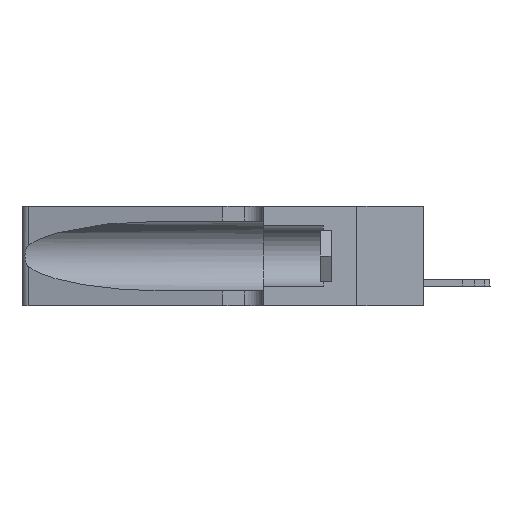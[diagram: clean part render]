
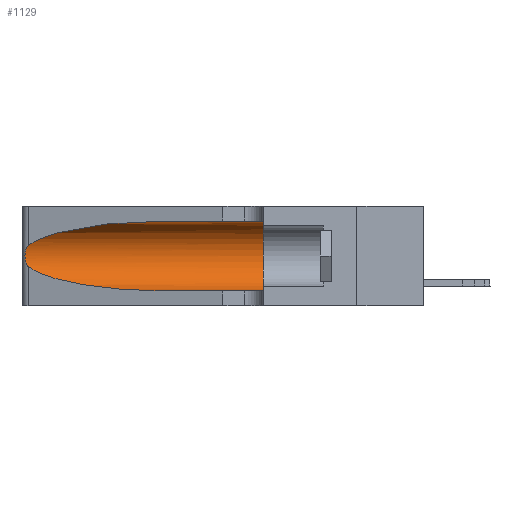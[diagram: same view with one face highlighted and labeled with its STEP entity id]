
A CAD part, left-side view. The second image highlights one B-rep face of the part: STEP entity #1129.
In plain terms, the highlighted cylindrical face has radius 3.308 mm (diameter 6.617 mm), a partial arc.
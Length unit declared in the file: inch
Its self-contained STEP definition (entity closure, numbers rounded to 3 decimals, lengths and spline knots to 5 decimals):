
#900 = CARTESIAN_POINT ( 'NONE',  ( 0.25487, 1.22718, 0.22369 ) ) ;
#940 = CARTESIAN_POINT ( 'NONE',  ( 0.1305, 1.61858, 0.185 ) ) ;
#1116 = CARTESIAN_POINT ( 'NONE',  ( 0.1305, 0.72297, 0.31525 ) ) ;
#1129 = ADVANCED_FACE ( 'NONE', ( #5063 ), #8446, .F. ) ;
#1958 = CARTESIAN_POINT ( 'NONE',  ( 0.25487, 1.22718, 0.14631 ) ) ;
#2099 = AXIS2_PLACEMENT_3D ( 'NONE', #940, #14384, #6208 ) ;
#2236 = EDGE_CURVE ( 'NONE', #19394, #9798, #2392, .T. ) ;
#2392 = B_SPLINE_CURVE_WITH_KNOTS ( 'NONE', 3,
 ( #900, #5565, #15732, #5869, #4059, #17380, #4411, #9474, #2837, #12801, #2765, #2911, #6093, #10994 ),
 .UNSPECIFIED., .F., .F.,
 ( 4, 2, 2, 2, 2, 2, 4 ),
 ( 0., 0.00027, 0.00053, 0.00107, 0.0016, 0.00187, 0.00214 ),
 .UNSPECIFIED. ) ;
#2627 = CARTESIAN_POINT ( 'NONE',  ( 0.1305, 0.72297, 0.31525 ) ) ;
#2703 = CARTESIAN_POINT ( 'NONE',  ( 0.25487, 1.22718, 0.22369 ) ) ;
#2765 = CARTESIAN_POINT ( 'NONE',  ( 0.25789, 1.23486, 0.15765 ) ) ;
#2837 = CARTESIAN_POINT ( 'NONE',  ( 0.26017, 1.23833, 0.17102 ) ) ;
#2911 = CARTESIAN_POINT ( 'NONE',  ( 0.25639, 1.23186, 0.15144 ) ) ;
#4059 = CARTESIAN_POINT ( 'NONE',  ( 0.25854, 1.2359, 0.20912 ) ) ;
#4278 = CARTESIAN_POINT ( 'NONE',  ( 0.2373, 1.15595, 0.28018 ) ) ;
#4411 = CARTESIAN_POINT ( 'NONE',  ( 0.26075, 1.23896, 0.19203 ) ) ;
#4442 = EDGE_CURVE ( 'NONE', #12166, #11646, #16792, .T. ) ;
#4621 = DIRECTION ( 'NONE',  ( 0., 1., 0. ) ) ;
#5063 = FACE_OUTER_BOUND ( 'NONE', #18109, .T. ) ;
#5565 = CARTESIAN_POINT ( 'NONE',  ( 0.25555, 1.22994, 0.2215 ) ) ;
#5667 = CARTESIAN_POINT ( 'NONE',  ( 0.25487, 1.22718, 0.14631 ) ) ;
#5869 = CARTESIAN_POINT ( 'NONE',  ( 0.25787, 1.23484, 0.2124 ) ) ;
#5948 = CARTESIAN_POINT ( 'NONE',  ( 0.18966, 0.96281, 0.31525 ) ) ;
#6093 = CARTESIAN_POINT ( 'NONE',  ( 0.25555, 1.22993, 0.14849 ) ) ;
#6208 = DIRECTION ( 'NONE',  ( 0., 0., -1. ) ) ;
#6311 = EDGE_CURVE ( 'NONE', #12266, #19394, #8343, .T. ) ;
#7285 = CARTESIAN_POINT ( 'NONE',  ( 0.1305, 0.35, 0.31525 ) ) ;
#7495 = CARTESIAN_POINT ( 'NONE',  ( 0.1305, 0.72297, 0.05475 ) ) ;
#7782 = CARTESIAN_POINT ( 'NONE',  ( 0.1305, 1.61858, 0.31525 ) ) ;
#8343 =( BOUNDED_CURVE ( )  B_SPLINE_CURVE ( 3, ( #2627, #5948, #4278, #2703 ),
 .UNSPECIFIED., .F., .T. ) 
 B_SPLINE_CURVE_WITH_KNOTS ( ( 4, 4 ),
 ( 1.5708, 2.84003 ),
 .UNSPECIFIED. ) 
 CURVE ( )  GEOMETRIC_REPRESENTATION_ITEM ( )  RATIONAL_B_SPLINE_CURVE ( ( 1., 0.87, 0.87, 1. ) ) 
 REPRESENTATION_ITEM ( '' )  );
#8446 = CYLINDRICAL_SURFACE ( 'NONE', #2099, 0.13025 ) ;
#9414 =( BOUNDED_CURVE ( )  B_SPLINE_CURVE ( 3, ( #5667, #12314, #10872, #7495 ),
 .UNSPECIFIED., .F., .T. ) 
 B_SPLINE_CURVE_WITH_KNOTS ( ( 4, 4 ),
 ( 3.44316, 4.71239 ),
 .UNSPECIFIED. ) 
 CURVE ( )  GEOMETRIC_REPRESENTATION_ITEM ( )  RATIONAL_B_SPLINE_CURVE ( ( 1., 0.87, 0.87, 1. ) ) 
 REPRESENTATION_ITEM ( '' )  );
#9474 = CARTESIAN_POINT ( 'NONE',  ( 0.26075, 1.23896, 0.178 ) ) ;
#9798 = VERTEX_POINT ( 'NONE', #1958 ) ;
#10486 = ORIENTED_EDGE ( 'NONE', *, *, #16818, .F. ) ;
#10689 = CARTESIAN_POINT ( 'NONE',  ( 0.1305, 1.61858, 0.05475 ) ) ;
#10872 = CARTESIAN_POINT ( 'NONE',  ( 0.18966, 0.96281, 0.05475 ) ) ;
#10994 = CARTESIAN_POINT ( 'NONE',  ( 0.25487, 1.22718, 0.14631 ) ) ;
#11200 = CARTESIAN_POINT ( 'NONE',  ( 0.25487, 1.22718, 0.22369 ) ) ;
#11646 = VERTEX_POINT ( 'NONE', #16860 ) ;
#11823 = VECTOR ( 'NONE', #12001, 39.37008 ) ;
#12001 = DIRECTION ( 'NONE',  ( 0., -1., 0. ) ) ;
#12166 = VERTEX_POINT ( 'NONE', #7285 ) ;
#12266 = VERTEX_POINT ( 'NONE', #1116 ) ;
#12294 = CARTESIAN_POINT ( 'NONE',  ( 0.1305, 0.35, 0.185 ) ) ;
#12314 = CARTESIAN_POINT ( 'NONE',  ( 0.2373, 1.15595, 0.08982 ) ) ;
#12671 = VECTOR ( 'NONE', #17974, 39.37008 ) ;
#12801 = CARTESIAN_POINT ( 'NONE',  ( 0.25856, 1.23593, 0.16098 ) ) ;
#13644 = ORIENTED_EDGE ( 'NONE', *, *, #17878, .T. ) ;
#13728 = ORIENTED_EDGE ( 'NONE', *, *, #16250, .T. ) ;
#14384 = DIRECTION ( 'NONE',  ( 0., -1., 0. ) ) ;
#15189 = CARTESIAN_POINT ( 'NONE',  ( 0.1305, 0.72297, 0.05475 ) ) ;
#15732 = CARTESIAN_POINT ( 'NONE',  ( 0.25639, 1.23184, 0.21858 ) ) ;
#15816 = VERTEX_POINT ( 'NONE', #15189 ) ;
#16250 = EDGE_CURVE ( 'NONE', #9798, #15816, #9414, .T. ) ;
#16486 = AXIS2_PLACEMENT_3D ( 'NONE', #12294, #4621, #20117 ) ;
#16792 = CIRCLE ( 'NONE', #16486, 0.13025 ) ;
#16818 = EDGE_CURVE ( 'NONE', #12266, #12166, #20891, .T. ) ;
#16860 = CARTESIAN_POINT ( 'NONE',  ( 0.1305, 0.35, 0.05475 ) ) ;
#17380 = CARTESIAN_POINT ( 'NONE',  ( 0.26018, 1.23835, 0.19895 ) ) ;
#17878 = EDGE_CURVE ( 'NONE', #15816, #11646, #20578, .T. ) ;
#17974 = DIRECTION ( 'NONE',  ( 0., -1., 0. ) ) ;
#18109 = EDGE_LOOP ( 'NONE', ( #19620, #19354, #13728, #13644, #18591, #10486 ) ) ;
#18591 = ORIENTED_EDGE ( 'NONE', *, *, #4442, .F. ) ;
#19354 = ORIENTED_EDGE ( 'NONE', *, *, #2236, .T. ) ;
#19394 = VERTEX_POINT ( 'NONE', #11200 ) ;
#19620 = ORIENTED_EDGE ( 'NONE', *, *, #6311, .T. ) ;
#20117 = DIRECTION ( 'NONE',  ( 0., 0., 1. ) ) ;
#20578 = LINE ( 'NONE', #10689, #11823 ) ;
#20891 = LINE ( 'NONE', #7782, #12671 ) ;
